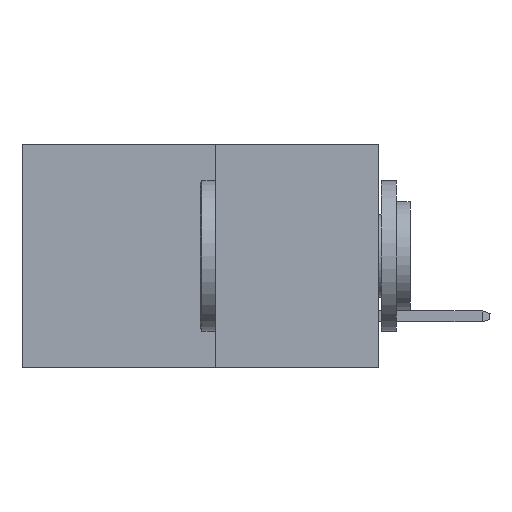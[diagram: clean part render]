
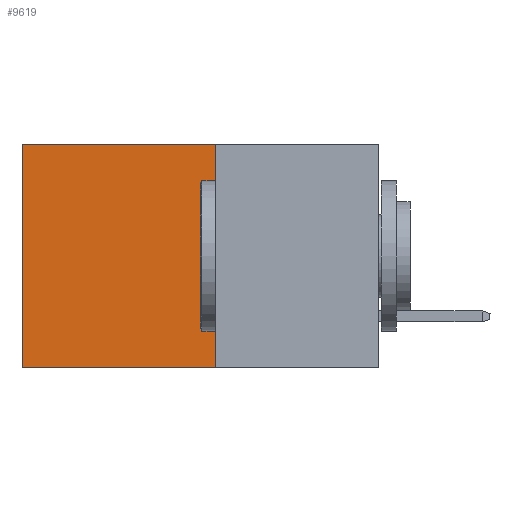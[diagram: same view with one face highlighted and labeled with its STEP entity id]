
A CAD part, left-side view. The second image highlights one B-rep face of the part: STEP entity #9619.
In plain terms, the highlighted planar face has unit normal (-1, 0, 0).
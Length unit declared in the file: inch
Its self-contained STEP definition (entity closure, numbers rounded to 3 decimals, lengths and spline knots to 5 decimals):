
#63 = LINE ( 'NONE', #4247, #5853 ) ;
#241 = ORIENTED_EDGE ( 'NONE', *, *, #6102, .F. ) ;
#452 = DIRECTION ( 'NONE',  ( 0., 0., -1. ) ) ;
#826 = VERTEX_POINT ( 'NONE', #9507 ) ;
#1004 = VERTEX_POINT ( 'NONE', #8049 ) ;
#1044 = AXIS2_PLACEMENT_3D ( 'NONE', #4127, #9341, #4893 ) ;
#1051 = VECTOR ( 'NONE', #7065, 39.37008 ) ;
#1070 = EDGE_CURVE ( 'NONE', #1081, #1004, #5754, .T. ) ;
#1081 = VERTEX_POINT ( 'NONE', #2083 ) ;
#1149 = VERTEX_POINT ( 'NONE', #9152 ) ;
#1175 = LINE ( 'NONE', #2302, #8897 ) ;
#1553 = LINE ( 'NONE', #9082, #1051 ) ;
#1710 = EDGE_CURVE ( 'NONE', #1081, #1149, #1553, .T. ) ;
#1896 = EDGE_CURVE ( 'NONE', #1149, #826, #1175, .T. ) ;
#2083 = CARTESIAN_POINT ( 'NONE',  ( 0.277, 0.27, 0. ) ) ;
#2302 = CARTESIAN_POINT ( 'NONE',  ( 0.277, 0.59, -0.37 ) ) ;
#3748 = VECTOR ( 'NONE', #7300, 39.37008 ) ;
#4127 = CARTESIAN_POINT ( 'NONE',  ( 0.277, 0.27, -0.37 ) ) ;
#4182 = ORIENTED_EDGE ( 'NONE', *, *, #1710, .T. ) ;
#4206 = DIRECTION ( 'NONE',  ( 0., 1., 0. ) ) ;
#4247 = CARTESIAN_POINT ( 'NONE',  ( 0.277, 0.27, -0.37 ) ) ;
#4893 = DIRECTION ( 'NONE',  ( 0., 0., -1. ) ) ;
#5073 = EDGE_LOOP ( 'NONE', ( #9225, #241, #6267, #4182 ) ) ;
#5754 = LINE ( 'NONE', #8250, #3748 ) ;
#5853 = VECTOR ( 'NONE', #4206, 39.37008 ) ;
#6102 = EDGE_CURVE ( 'NONE', #1004, #826, #63, .T. ) ;
#6267 = ORIENTED_EDGE ( 'NONE', *, *, #1070, .F. ) ;
#6814 = FACE_OUTER_BOUND ( 'NONE', #5073, .T. ) ;
#7065 = DIRECTION ( 'NONE',  ( 0., 1., 0. ) ) ;
#7300 = DIRECTION ( 'NONE',  ( 0., 0., -1. ) ) ;
#8049 = CARTESIAN_POINT ( 'NONE',  ( 0.277, 0.27, -0.37 ) ) ;
#8250 = CARTESIAN_POINT ( 'NONE',  ( 0.277, 0.27, -0.37 ) ) ;
#8551 = PLANE ( 'NONE',  #1044 ) ;
#8897 = VECTOR ( 'NONE', #452, 39.37008 ) ;
#9082 = CARTESIAN_POINT ( 'NONE',  ( 0.277, 0.27, 0. ) ) ;
#9152 = CARTESIAN_POINT ( 'NONE',  ( 0.277, 0.59, 0. ) ) ;
#9225 = ORIENTED_EDGE ( 'NONE', *, *, #1896, .T. ) ;
#9341 = DIRECTION ( 'NONE',  ( 1., 0., 0. ) ) ;
#9507 = CARTESIAN_POINT ( 'NONE',  ( 0.277, 0.59, -0.37 ) ) ;
#9619 = ADVANCED_FACE ( 'NONE', ( #6814 ), #8551, .F. ) ;
